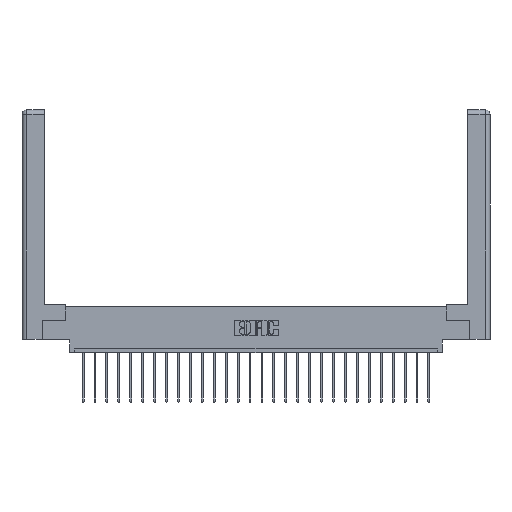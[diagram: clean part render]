
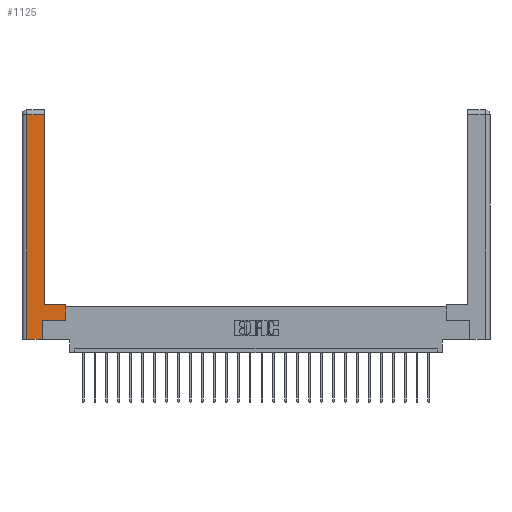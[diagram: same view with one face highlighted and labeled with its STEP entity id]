
A CAD part, top view. The second image highlights one B-rep face of the part: STEP entity #1125.
In plain terms, the highlighted planar face has unit normal (0, 0, 1).
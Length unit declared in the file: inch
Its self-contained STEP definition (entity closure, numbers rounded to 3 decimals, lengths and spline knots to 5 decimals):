
#7 = LINE ( 'NONE', #15010, #15858 ) ;
#322 = CARTESIAN_POINT ( 'NONE',  ( 0.0615, 2.94, 0. ) ) ;
#336 = DIRECTION ( 'NONE',  ( -1., 0., 0. ) ) ;
#637 = DIRECTION ( 'NONE',  ( 0., -1., 0. ) ) ;
#751 = DIRECTION ( 'NONE',  ( 0., 1., 0. ) ) ;
#815 = EDGE_CURVE ( 'NONE', #14103, #20358, #6549, .T. ) ;
#832 = ORIENTED_EDGE ( 'NONE', *, *, #22471, .T. ) ;
#1125 = ADVANCED_FACE ( 'NONE', ( #1399 ), #13862, .F. ) ;
#1321 = DIRECTION ( 'NONE',  ( 0., 0., -1. ) ) ;
#1399 = FACE_OUTER_BOUND ( 'NONE', #8640, .T. ) ;
#1491 = CARTESIAN_POINT ( 'NONE',  ( 0., 0., 0. ) ) ;
#2105 = ORIENTED_EDGE ( 'NONE', *, *, #19622, .T. ) ;
#2546 = VECTOR ( 'NONE', #637, 39.37008 ) ;
#3604 = DIRECTION ( 'NONE',  ( -1., 0., 0. ) ) ;
#4432 = EDGE_CURVE ( 'NONE', #16770, #11648, #13870, .T. ) ;
#5013 = CARTESIAN_POINT ( 'NONE',  ( 0.0615, 0., 0. ) ) ;
#5062 = LINE ( 'NONE', #9507, #15412 ) ;
#6549 = LINE ( 'NONE', #24316, #10772 ) ;
#7603 = VECTOR ( 'NONE', #336, 39.37008 ) ;
#8640 = EDGE_LOOP ( 'NONE', ( #18307, #832, #21542, #9884, #22528, #12948, #2105, #9583 ) ) ;
#8666 = CARTESIAN_POINT ( 'NONE',  ( 0.0615, 0., 0. ) ) ;
#8760 = VERTEX_POINT ( 'NONE', #15003 ) ;
#9214 = DIRECTION ( 'NONE',  ( 1., 0., 0. ) ) ;
#9507 = CARTESIAN_POINT ( 'NONE',  ( 0.265, 0., 0. ) ) ;
#9583 = ORIENTED_EDGE ( 'NONE', *, *, #21633, .T. ) ;
#9884 = ORIENTED_EDGE ( 'NONE', *, *, #21550, .T. ) ;
#10772 = VECTOR ( 'NONE', #26403, 39.37008 ) ;
#11648 = VERTEX_POINT ( 'NONE', #5013 ) ;
#12228 = LINE ( 'NONE', #19335, #22813 ) ;
#12830 = VERTEX_POINT ( 'NONE', #20078 ) ;
#12948 = ORIENTED_EDGE ( 'NONE', *, *, #19074, .T. ) ;
#13463 = LINE ( 'NONE', #20793, #7603 ) ;
#13497 = DIRECTION ( 'NONE',  ( -1., 0., 0. ) ) ;
#13862 = PLANE ( 'NONE',  #17915 ) ;
#13870 = LINE ( 'NONE', #8666, #2546 ) ;
#13882 = CARTESIAN_POINT ( 'NONE',  ( 0.295, 2.94, 0. ) ) ;
#14103 = VERTEX_POINT ( 'NONE', #26335 ) ;
#14776 = VECTOR ( 'NONE', #18906, 39.37008 ) ;
#14973 = EDGE_CURVE ( 'NONE', #8760, #12830, #21499, .T. ) ;
#15003 = CARTESIAN_POINT ( 'NONE',  ( 0.265, 0., 0. ) ) ;
#15010 = CARTESIAN_POINT ( 'NONE',  ( 0.565, 0.245, 0. ) ) ;
#15412 = VECTOR ( 'NONE', #25097, 39.37008 ) ;
#15858 = VECTOR ( 'NONE', #9214, 39.37008 ) ;
#16770 = VERTEX_POINT ( 'NONE', #322 ) ;
#17259 = VERTEX_POINT ( 'NONE', #25330 ) ;
#17915 = AXIS2_PLACEMENT_3D ( 'NONE', #1491, #1321, #13497 ) ;
#18307 = ORIENTED_EDGE ( 'NONE', *, *, #815, .T. ) ;
#18312 = VECTOR ( 'NONE', #3604, 39.37008 ) ;
#18419 = VERTEX_POINT ( 'NONE', #22545 ) ;
#18906 = DIRECTION ( 'NONE',  ( 0., 1., 0. ) ) ;
#19000 = CARTESIAN_POINT ( 'NONE',  ( 0.265, 0.245, 0. ) ) ;
#19074 = EDGE_CURVE ( 'NONE', #12830, #17259, #7, .T. ) ;
#19335 = CARTESIAN_POINT ( 'NONE',  ( 0.565, 0.45, 0. ) ) ;
#19622 = EDGE_CURVE ( 'NONE', #17259, #18419, #12228, .T. ) ;
#20078 = CARTESIAN_POINT ( 'NONE',  ( 0.265, 0.245, 0. ) ) ;
#20358 = VERTEX_POINT ( 'NONE', #13882 ) ;
#20793 = CARTESIAN_POINT ( 'NONE',  ( 0.0615, 2.94, 0. ) ) ;
#21499 = LINE ( 'NONE', #19000, #14776 ) ;
#21542 = ORIENTED_EDGE ( 'NONE', *, *, #4432, .T. ) ;
#21550 = EDGE_CURVE ( 'NONE', #11648, #8760, #5062, .T. ) ;
#21633 = EDGE_CURVE ( 'NONE', #18419, #14103, #23057, .T. ) ;
#22471 = EDGE_CURVE ( 'NONE', #20358, #16770, #13463, .T. ) ;
#22528 = ORIENTED_EDGE ( 'NONE', *, *, #14973, .T. ) ;
#22545 = CARTESIAN_POINT ( 'NONE',  ( 0.565, 0.45, 0. ) ) ;
#22813 = VECTOR ( 'NONE', #751, 39.37008 ) ;
#23057 = LINE ( 'NONE', #26324, #18312 ) ;
#24316 = CARTESIAN_POINT ( 'NONE',  ( 0.295, 3., 0. ) ) ;
#25097 = DIRECTION ( 'NONE',  ( 1., 0., 0. ) ) ;
#25330 = CARTESIAN_POINT ( 'NONE',  ( 0.565, 0.245, 0. ) ) ;
#26324 = CARTESIAN_POINT ( 'NONE',  ( 0.295, 0.45, 0. ) ) ;
#26335 = CARTESIAN_POINT ( 'NONE',  ( 0.295, 0.45, 0. ) ) ;
#26403 = DIRECTION ( 'NONE',  ( 0., 1., 0. ) ) ;
